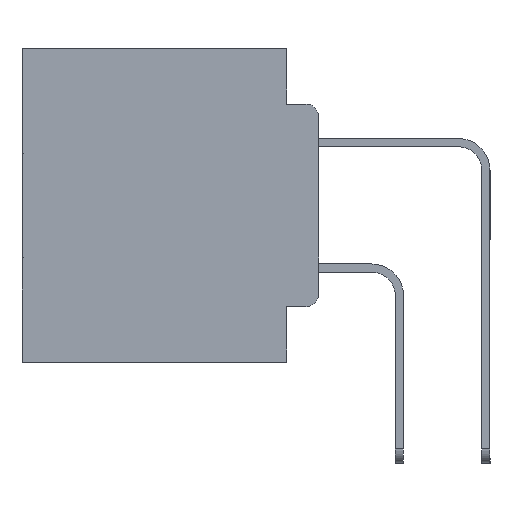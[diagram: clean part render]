
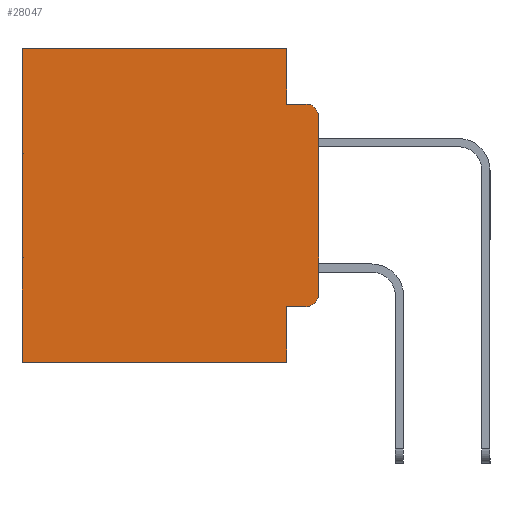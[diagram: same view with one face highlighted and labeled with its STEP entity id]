
A CAD part, left-side view. The second image highlights one B-rep face of the part: STEP entity #28047.
In plain terms, the highlighted planar face has unit normal (-1, 0, 0).
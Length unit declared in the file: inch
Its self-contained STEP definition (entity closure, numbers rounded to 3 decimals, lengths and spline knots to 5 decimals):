
#50 = ORIENTED_EDGE ( 'NONE', *, *, #23555, .F. ) ;
#178 = EDGE_CURVE ( 'NONE', #14492, #9784, #21803, .T. ) ;
#303 = DIRECTION ( 'NONE',  ( 0., 0., -1. ) ) ;
#512 = LINE ( 'NONE', #22975, #20639 ) ;
#1230 = LINE ( 'NONE', #22000, #13436 ) ;
#1340 = DIRECTION ( 'NONE',  ( 0., -1., 0. ) ) ;
#1761 = CARTESIAN_POINT ( 'NONE',  ( 0.298, 0.051, 0. ) ) ;
#2169 = CARTESIAN_POINT ( 'NONE',  ( 0.298, 0., -0.3915 ) ) ;
#2670 = AXIS2_PLACEMENT_3D ( 'NONE', #9379, #26214, #11795 ) ;
#2877 = VECTOR ( 'NONE', #26052, 39.37008 ) ;
#3160 = VERTEX_POINT ( 'NONE', #27007 ) ;
#4154 = CARTESIAN_POINT ( 'NONE',  ( 0.298, 0., 0. ) ) ;
#4364 = CARTESIAN_POINT ( 'NONE',  ( 0.298, 0.02, -0.4115 ) ) ;
#4634 = CARTESIAN_POINT ( 'NONE',  ( 0.298, 0.02, -0.0885 ) ) ;
#5048 = DIRECTION ( 'NONE',  ( 0., 1., 0. ) ) ;
#6170 = DIRECTION ( 'NONE',  ( 0., 0., -1. ) ) ;
#7098 = CARTESIAN_POINT ( 'NONE',  ( 0.298, 0.051, 0. ) ) ;
#7240 = EDGE_LOOP ( 'NONE', ( #17537, #12632, #19060, #9231, #28388, #23585, #11501, #50, #13803, #8094 ) ) ;
#7286 = LINE ( 'NONE', #18310, #14527 ) ;
#8094 = ORIENTED_EDGE ( 'NONE', *, *, #15486, .T. ) ;
#8342 = DIRECTION ( 'NONE',  ( -1., 0., 0. ) ) ;
#8379 = CARTESIAN_POINT ( 'NONE',  ( 0.298, 0.02, -0.1085 ) ) ;
#8383 = EDGE_CURVE ( 'NONE', #14492, #20530, #512, .T. ) ;
#9176 = VECTOR ( 'NONE', #19180, 39.37008 ) ;
#9231 = ORIENTED_EDGE ( 'NONE', *, *, #26735, .F. ) ;
#9379 = CARTESIAN_POINT ( 'NONE',  ( 0.298, 0.02, -0.3915 ) ) ;
#9784 = VERTEX_POINT ( 'NONE', #4634 ) ;
#10626 = VECTOR ( 'NONE', #303, 39.37008 ) ;
#11138 = DIRECTION ( 'NONE',  ( 0., -1., 0. ) ) ;
#11501 = ORIENTED_EDGE ( 'NONE', *, *, #22377, .F. ) ;
#11795 = DIRECTION ( 'NONE',  ( 0., 0., -1. ) ) ;
#11901 = LINE ( 'NONE', #20845, #23987 ) ;
#12406 = VERTEX_POINT ( 'NONE', #18356 ) ;
#12540 = VERTEX_POINT ( 'NONE', #4364 ) ;
#12603 = CARTESIAN_POINT ( 'NONE',  ( 0.298, 0., -0.1085 ) ) ;
#12632 = ORIENTED_EDGE ( 'NONE', *, *, #178, .T. ) ;
#13374 = DIRECTION ( 'NONE',  ( 0., 0., -1. ) ) ;
#13403 = LINE ( 'NONE', #4154, #26178 ) ;
#13436 = VECTOR ( 'NONE', #5048, 39.37008 ) ;
#13803 = ORIENTED_EDGE ( 'NONE', *, *, #17098, .T. ) ;
#14492 = VERTEX_POINT ( 'NONE', #12603 ) ;
#14527 = VECTOR ( 'NONE', #1340, 39.37008 ) ;
#14911 = CARTESIAN_POINT ( 'NONE',  ( 0.298, 0.473, 0. ) ) ;
#15140 = CARTESIAN_POINT ( 'NONE',  ( 0.298, 0.051, -0.5 ) ) ;
#15486 = EDGE_CURVE ( 'NONE', #12540, #20530, #19583, .T. ) ;
#17098 = EDGE_CURVE ( 'NONE', #12406, #12540, #11901, .T. ) ;
#17184 = VERTEX_POINT ( 'NONE', #1761 ) ;
#17438 = VERTEX_POINT ( 'NONE', #29154 ) ;
#17537 = ORIENTED_EDGE ( 'NONE', *, *, #8383, .F. ) ;
#18310 = CARTESIAN_POINT ( 'NONE',  ( 0.298, 0.051, -0.0885 ) ) ;
#18356 = CARTESIAN_POINT ( 'NONE',  ( 0.298, 0.051, -0.4115 ) ) ;
#18694 = CARTESIAN_POINT ( 'NONE',  ( 0.298, 0.473, 0. ) ) ;
#18762 = AXIS2_PLACEMENT_3D ( 'NONE', #20521, #27727, #13374 ) ;
#19060 = ORIENTED_EDGE ( 'NONE', *, *, #29899, .F. ) ;
#19077 = VERTEX_POINT ( 'NONE', #18694 ) ;
#19180 = DIRECTION ( 'NONE',  ( 0., 0., -1. ) ) ;
#19583 = CIRCLE ( 'NONE', #2670, 0.02 ) ;
#20521 = CARTESIAN_POINT ( 'NONE',  ( 0.298, 0., 0. ) ) ;
#20530 = VERTEX_POINT ( 'NONE', #2169 ) ;
#20639 = VECTOR ( 'NONE', #25333, 39.37008 ) ;
#20845 = CARTESIAN_POINT ( 'NONE',  ( 0.298, 0.051, -0.4115 ) ) ;
#21129 = DIRECTION ( 'NONE',  ( 0., 1., 0. ) ) ;
#21803 = CIRCLE ( 'NONE', #23275, 0.02 ) ;
#22000 = CARTESIAN_POINT ( 'NONE',  ( 0.298, 0., -0.5 ) ) ;
#22238 = LINE ( 'NONE', #23665, #2877 ) ;
#22377 = EDGE_CURVE ( 'NONE', #28523, #17438, #1230, .T. ) ;
#22779 = EDGE_CURVE ( 'NONE', #17184, #19077, #13403, .T. ) ;
#22858 = PLANE ( 'NONE',  #18762 ) ;
#22975 = CARTESIAN_POINT ( 'NONE',  ( 0.298, 0., 0. ) ) ;
#23275 = AXIS2_PLACEMENT_3D ( 'NONE', #8379, #8342, #6170 ) ;
#23309 = FACE_OUTER_BOUND ( 'NONE', #7240, .T. ) ;
#23555 = EDGE_CURVE ( 'NONE', #12406, #28523, #29083, .T. ) ;
#23585 = ORIENTED_EDGE ( 'NONE', *, *, #25150, .T. ) ;
#23665 = CARTESIAN_POINT ( 'NONE',  ( 0.298, 0.051, 0. ) ) ;
#23987 = VECTOR ( 'NONE', #11138, 39.37008 ) ;
#25150 = EDGE_CURVE ( 'NONE', #19077, #17438, #29031, .T. ) ;
#25333 = DIRECTION ( 'NONE',  ( 0., 0., -1. ) ) ;
#26052 = DIRECTION ( 'NONE',  ( 0., 0., -1. ) ) ;
#26178 = VECTOR ( 'NONE', #21129, 39.37008 ) ;
#26214 = DIRECTION ( 'NONE',  ( -1., 0., 0. ) ) ;
#26735 = EDGE_CURVE ( 'NONE', #17184, #3160, #22238, .T. ) ;
#27007 = CARTESIAN_POINT ( 'NONE',  ( 0.298, 0.051, -0.0885 ) ) ;
#27727 = DIRECTION ( 'NONE',  ( 1., 0., 0. ) ) ;
#28047 = ADVANCED_FACE ( 'NONE', ( #23309 ), #22858, .F. ) ;
#28388 = ORIENTED_EDGE ( 'NONE', *, *, #22779, .T. ) ;
#28523 = VERTEX_POINT ( 'NONE', #15140 ) ;
#29031 = LINE ( 'NONE', #14911, #10626 ) ;
#29083 = LINE ( 'NONE', #7098, #9176 ) ;
#29154 = CARTESIAN_POINT ( 'NONE',  ( 0.298, 0.473, -0.5 ) ) ;
#29899 = EDGE_CURVE ( 'NONE', #3160, #9784, #7286, .T. ) ;
